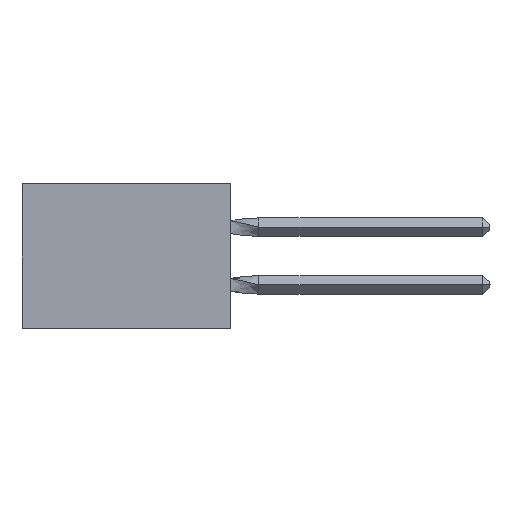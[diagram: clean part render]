
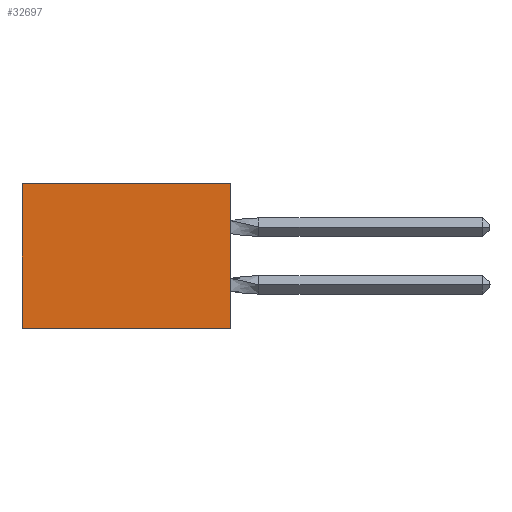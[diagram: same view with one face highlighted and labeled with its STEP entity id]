
A CAD part, left-side view. The second image highlights one B-rep face of the part: STEP entity #32697.
In plain terms, the highlighted planar face has unit normal (-1, 0, 0).
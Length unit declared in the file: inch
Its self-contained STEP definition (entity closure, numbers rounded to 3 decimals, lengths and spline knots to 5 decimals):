
#1346 = PLANE ( 'NONE',  #24355 ) ;
#2845 = CARTESIAN_POINT ( 'NONE',  ( 0.305, 0., -0.5 ) ) ;
#3356 = EDGE_CURVE ( 'NONE', #26461, #9771, #16735, .T. ) ;
#3934 = VERTEX_POINT ( 'NONE', #15238 ) ;
#4614 = EDGE_CURVE ( 'NONE', #30281, #26461, #23041, .T. ) ;
#5683 = DIRECTION ( 'NONE',  ( 0., 0., -1. ) ) ;
#5905 = ORIENTED_EDGE ( 'NONE', *, *, #11359, .F. ) ;
#6699 = CARTESIAN_POINT ( 'NONE',  ( 0.305, 0., -0.5 ) ) ;
#9771 = VERTEX_POINT ( 'NONE', #18808 ) ;
#11359 = EDGE_CURVE ( 'NONE', #30281, #3934, #16575, .T. ) ;
#12230 = EDGE_LOOP ( 'NONE', ( #14899, #16799, #5905, #15033 ) ) ;
#14899 = ORIENTED_EDGE ( 'NONE', *, *, #3356, .T. ) ;
#15033 = ORIENTED_EDGE ( 'NONE', *, *, #4614, .T. ) ;
#15238 = CARTESIAN_POINT ( 'NONE',  ( 0.305, 0., -0.5 ) ) ;
#15493 = DIRECTION ( 'NONE',  ( 0., 0., -1. ) ) ;
#15884 = CARTESIAN_POINT ( 'NONE',  ( 0.305, 0., 0. ) ) ;
#16575 = LINE ( 'NONE', #2845, #28484 ) ;
#16735 = LINE ( 'NONE', #28486, #20162 ) ;
#16799 = ORIENTED_EDGE ( 'NONE', *, *, #26207, .F. ) ;
#17249 = FACE_OUTER_BOUND ( 'NONE', #12230, .T. ) ;
#18808 = CARTESIAN_POINT ( 'NONE',  ( 0.305, 0.72, -0.5 ) ) ;
#19616 = VECTOR ( 'NONE', #29590, 39.37008 ) ;
#20048 = DIRECTION ( 'NONE',  ( 0., 0., -1. ) ) ;
#20162 = VECTOR ( 'NONE', #15493, 39.37008 ) ;
#21985 = CARTESIAN_POINT ( 'NONE',  ( 0.305, 0., -0.5 ) ) ;
#23041 = LINE ( 'NONE', #15884, #19616 ) ;
#24355 = AXIS2_PLACEMENT_3D ( 'NONE', #6699, #31473, #20048 ) ;
#25339 = VECTOR ( 'NONE', #29960, 39.37008 ) ;
#26207 = EDGE_CURVE ( 'NONE', #3934, #9771, #32143, .T. ) ;
#26461 = VERTEX_POINT ( 'NONE', #31902 ) ;
#28484 = VECTOR ( 'NONE', #5683, 39.37008 ) ;
#28486 = CARTESIAN_POINT ( 'NONE',  ( 0.305, 0.72, -0.5 ) ) ;
#29590 = DIRECTION ( 'NONE',  ( 0., 1., 0. ) ) ;
#29960 = DIRECTION ( 'NONE',  ( 0., 1., 0. ) ) ;
#30281 = VERTEX_POINT ( 'NONE', #32055 ) ;
#31473 = DIRECTION ( 'NONE',  ( 1., 0., 0. ) ) ;
#31902 = CARTESIAN_POINT ( 'NONE',  ( 0.305, 0.72, 0. ) ) ;
#32055 = CARTESIAN_POINT ( 'NONE',  ( 0.305, 0., 0. ) ) ;
#32143 = LINE ( 'NONE', #21985, #25339 ) ;
#32697 = ADVANCED_FACE ( 'NONE', ( #17249 ), #1346, .F. ) ;
